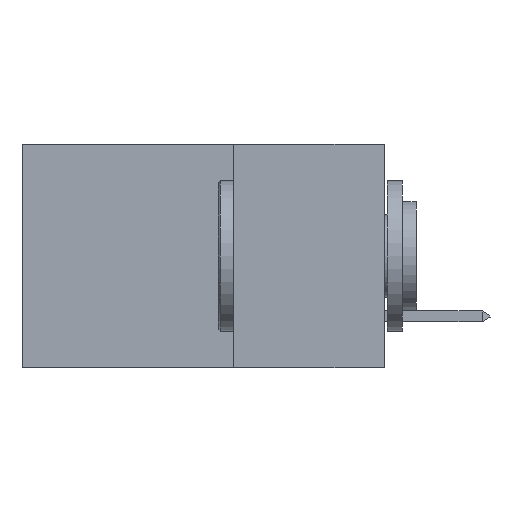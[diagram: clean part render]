
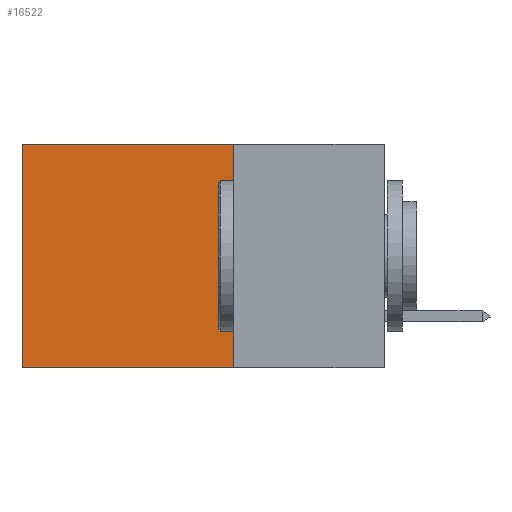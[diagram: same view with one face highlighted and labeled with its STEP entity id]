
A CAD part, left-side view. The second image highlights one B-rep face of the part: STEP entity #16522.
In plain terms, the highlighted planar face has unit normal (-1, 0, 0).
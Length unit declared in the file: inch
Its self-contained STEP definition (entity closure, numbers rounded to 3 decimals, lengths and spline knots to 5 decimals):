
#1865 = VERTEX_POINT ( 'NONE', #29900 ) ;
#2229 = FACE_OUTER_BOUND ( 'NONE', #5664, .T. ) ;
#4488 = VECTOR ( 'NONE', #11084, 39.37008 ) ;
#5309 = EDGE_CURVE ( 'NONE', #7373, #20002, #34540, .T. ) ;
#5664 = EDGE_LOOP ( 'NONE', ( #36157, #13614, #18432, #15516 ) ) ;
#7373 = VERTEX_POINT ( 'NONE', #9941 ) ;
#7943 = DIRECTION ( 'NONE',  ( 0., 1., 0. ) ) ;
#8209 = CARTESIAN_POINT ( 'NONE',  ( 0.2875, 0.6, 0. ) ) ;
#8236 = VERTEX_POINT ( 'NONE', #32185 ) ;
#8937 = CARTESIAN_POINT ( 'NONE',  ( 0.2875, 0.6, -0.37 ) ) ;
#9941 = CARTESIAN_POINT ( 'NONE',  ( 0.2875, 0.25, -0.37 ) ) ;
#9973 = EDGE_CURVE ( 'NONE', #8236, #20002, #27550, .T. ) ;
#11084 = DIRECTION ( 'NONE',  ( 0., 0., -1. ) ) ;
#11331 = DIRECTION ( 'NONE',  ( 1., 0., 0. ) ) ;
#12437 = DIRECTION ( 'NONE',  ( 0., 1., 0. ) ) ;
#13614 = ORIENTED_EDGE ( 'NONE', *, *, #5309, .F. ) ;
#14804 = VECTOR ( 'NONE', #7943, 39.37008 ) ;
#15516 = ORIENTED_EDGE ( 'NONE', *, *, #36701, .T. ) ;
#16462 = CARTESIAN_POINT ( 'NONE',  ( 0.2875, 0.25, 0. ) ) ;
#16522 = ADVANCED_FACE ( 'NONE', ( #2229 ), #28683, .F. ) ;
#18432 = ORIENTED_EDGE ( 'NONE', *, *, #30273, .F. ) ;
#18976 = DIRECTION ( 'NONE',  ( 0., 0., -1. ) ) ;
#19962 = CARTESIAN_POINT ( 'NONE',  ( 0.2875, 0.25, 0. ) ) ;
#20002 = VERTEX_POINT ( 'NONE', #8937 ) ;
#22542 = LINE ( 'NONE', #16462, #14804 ) ;
#24735 = LINE ( 'NONE', #33346, #32385 ) ;
#25737 = AXIS2_PLACEMENT_3D ( 'NONE', #19962, #11331, #31568 ) ;
#27550 = LINE ( 'NONE', #8209, #4488 ) ;
#28683 = PLANE ( 'NONE',  #25737 ) ;
#29900 = CARTESIAN_POINT ( 'NONE',  ( 0.2875, 0.25, 0. ) ) ;
#30273 = EDGE_CURVE ( 'NONE', #1865, #7373, #24735, .T. ) ;
#31568 = DIRECTION ( 'NONE',  ( 0., 0., -1. ) ) ;
#32185 = CARTESIAN_POINT ( 'NONE',  ( 0.2875, 0.6, 0. ) ) ;
#32385 = VECTOR ( 'NONE', #18976, 39.37008 ) ;
#33346 = CARTESIAN_POINT ( 'NONE',  ( 0.2875, 0.25, 0. ) ) ;
#33652 = VECTOR ( 'NONE', #12437, 39.37008 ) ;
#34540 = LINE ( 'NONE', #35508, #33652 ) ;
#35508 = CARTESIAN_POINT ( 'NONE',  ( 0.2875, 0.25, -0.37 ) ) ;
#36157 = ORIENTED_EDGE ( 'NONE', *, *, #9973, .T. ) ;
#36701 = EDGE_CURVE ( 'NONE', #1865, #8236, #22542, .T. ) ;
